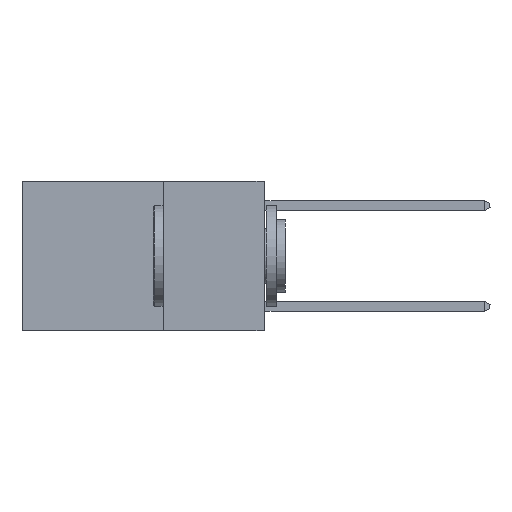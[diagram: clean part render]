
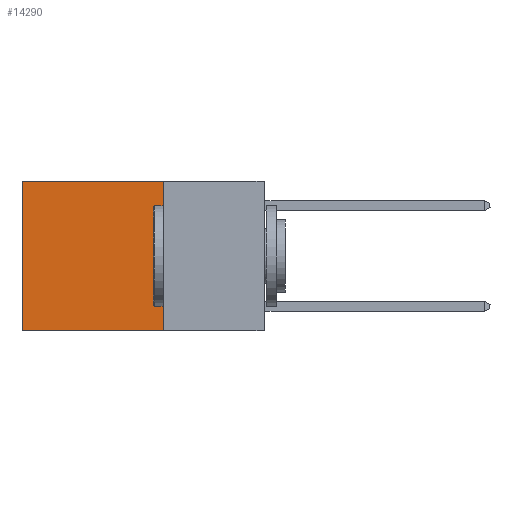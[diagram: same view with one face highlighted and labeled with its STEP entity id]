
A CAD part, left-side view. The second image highlights one B-rep face of the part: STEP entity #14290.
In plain terms, the highlighted planar face has unit normal (-1, 0, 0).
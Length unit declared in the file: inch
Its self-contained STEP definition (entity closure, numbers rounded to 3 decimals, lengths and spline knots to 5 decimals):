
#178 = CARTESIAN_POINT ( 'NONE',  ( 0.2625, 0.25, -0.37 ) ) ;
#995 = LINE ( 'NONE', #12256, #24258 ) ;
#1129 = DIRECTION ( 'NONE',  ( 0., 0., -1. ) ) ;
#1281 = FACE_OUTER_BOUND ( 'NONE', #28361, .T. ) ;
#1664 = CARTESIAN_POINT ( 'NONE',  ( 0.2625, 0.25, 0. ) ) ;
#2450 = EDGE_CURVE ( 'NONE', #10291, #12830, #2623, .T. ) ;
#2623 = LINE ( 'NONE', #18466, #23224 ) ;
#2968 = VECTOR ( 'NONE', #21417, 39.37008 ) ;
#3515 = EDGE_CURVE ( 'NONE', #9280, #12830, #995, .T. ) ;
#4932 = ORIENTED_EDGE ( 'NONE', *, *, #9879, .F. ) ;
#6009 = VERTEX_POINT ( 'NONE', #1664 ) ;
#7086 = LINE ( 'NONE', #25856, #2968 ) ;
#7821 = ORIENTED_EDGE ( 'NONE', *, *, #3515, .T. ) ;
#7831 = PLANE ( 'NONE',  #16106 ) ;
#8642 = LINE ( 'NONE', #11840, #21658 ) ;
#9280 = VERTEX_POINT ( 'NONE', #27710 ) ;
#9879 = EDGE_CURVE ( 'NONE', #6009, #10291, #8642, .T. ) ;
#10291 = VERTEX_POINT ( 'NONE', #178 ) ;
#11840 = CARTESIAN_POINT ( 'NONE',  ( 0.2625, 0.25, 0. ) ) ;
#12256 = CARTESIAN_POINT ( 'NONE',  ( 0.2625, 0.6, 0. ) ) ;
#12389 = CARTESIAN_POINT ( 'NONE',  ( 0.2625, 0.25, 0. ) ) ;
#12813 = ORIENTED_EDGE ( 'NONE', *, *, #13627, .T. ) ;
#12830 = VERTEX_POINT ( 'NONE', #22914 ) ;
#13627 = EDGE_CURVE ( 'NONE', #6009, #9280, #7086, .T. ) ;
#14290 = ADVANCED_FACE ( 'NONE', ( #1281 ), #7831, .F. ) ;
#16106 = AXIS2_PLACEMENT_3D ( 'NONE', #12389, #19088, #1129 ) ;
#18466 = CARTESIAN_POINT ( 'NONE',  ( 0.2625, 0.25, -0.37 ) ) ;
#19088 = DIRECTION ( 'NONE',  ( 1., 0., 0. ) ) ;
#21414 = DIRECTION ( 'NONE',  ( 0., 0., -1. ) ) ;
#21417 = DIRECTION ( 'NONE',  ( 0., 1., 0. ) ) ;
#21658 = VECTOR ( 'NONE', #21414, 39.37008 ) ;
#22914 = CARTESIAN_POINT ( 'NONE',  ( 0.2625, 0.6, -0.37 ) ) ;
#23224 = VECTOR ( 'NONE', #27763, 39.37008 ) ;
#24258 = VECTOR ( 'NONE', #26596, 39.37008 ) ;
#25431 = ORIENTED_EDGE ( 'NONE', *, *, #2450, .F. ) ;
#25856 = CARTESIAN_POINT ( 'NONE',  ( 0.2625, 0.25, 0. ) ) ;
#26596 = DIRECTION ( 'NONE',  ( 0., 0., -1. ) ) ;
#27710 = CARTESIAN_POINT ( 'NONE',  ( 0.2625, 0.6, 0. ) ) ;
#27763 = DIRECTION ( 'NONE',  ( 0., 1., 0. ) ) ;
#28361 = EDGE_LOOP ( 'NONE', ( #7821, #25431, #4932, #12813 ) ) ;
